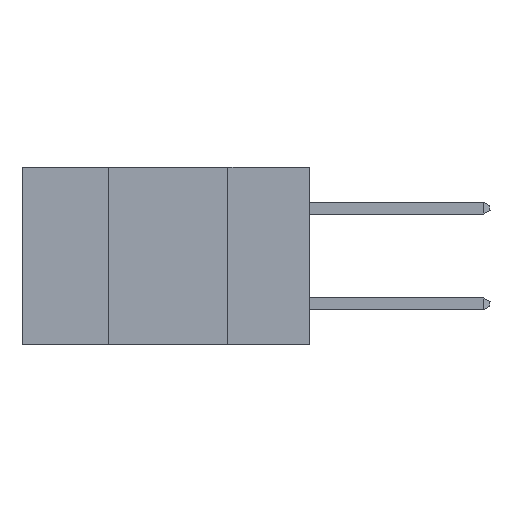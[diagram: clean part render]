
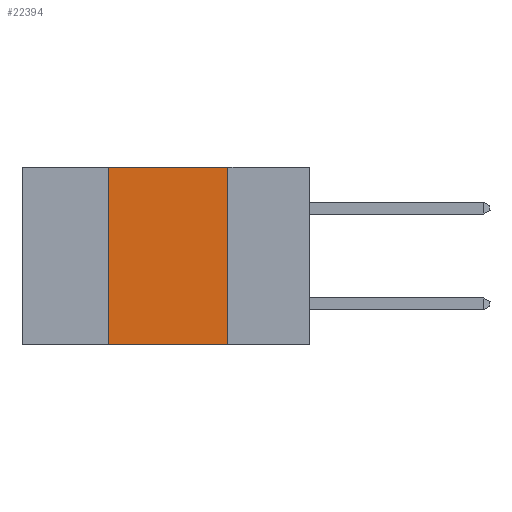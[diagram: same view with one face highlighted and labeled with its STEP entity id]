
A CAD part, left-side view. The second image highlights one B-rep face of the part: STEP entity #22394.
In plain terms, the highlighted planar face has unit normal (-1, 0, 0).
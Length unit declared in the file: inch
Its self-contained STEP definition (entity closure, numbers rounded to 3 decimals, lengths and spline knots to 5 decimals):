
#157 = LINE ( 'NONE', #28019, #7155 ) ;
#649 = EDGE_CURVE ( 'NONE', #26703, #19103, #25296, .T. ) ;
#2117 = DIRECTION ( 'NONE',  ( 0., 0., -1. ) ) ;
#2848 = LINE ( 'NONE', #33479, #21224 ) ;
#3149 = VERTEX_POINT ( 'NONE', #25572 ) ;
#4349 = DIRECTION ( 'NONE',  ( 0., -1., 0. ) ) ;
#6671 = CARTESIAN_POINT ( 'NONE',  ( 0., 0.6, -0.37 ) ) ;
#7155 = VECTOR ( 'NONE', #7980, 39.37008 ) ;
#7980 = DIRECTION ( 'NONE',  ( 0., 0., 1. ) ) ;
#8028 = FACE_OUTER_BOUND ( 'NONE', #17641, .T. ) ;
#10163 = PLANE ( 'NONE',  #22020 ) ;
#14916 = ORIENTED_EDGE ( 'NONE', *, *, #29927, .T. ) ;
#16187 = LINE ( 'NONE', #6671, #20147 ) ;
#17641 = EDGE_LOOP ( 'NONE', ( #25315, #28870, #25459, #14916 ) ) ;
#17831 = VECTOR ( 'NONE', #28814, 39.37008 ) ;
#18971 = CARTESIAN_POINT ( 'NONE',  ( 0., 0.6, 0. ) ) ;
#19103 = VERTEX_POINT ( 'NONE', #31976 ) ;
#19559 = DIRECTION ( 'NONE',  ( 0., 0., -1. ) ) ;
#20147 = VECTOR ( 'NONE', #4349, 39.37008 ) ;
#21224 = VECTOR ( 'NONE', #19559, 39.37008 ) ;
#22020 = AXIS2_PLACEMENT_3D ( 'NONE', #18971, #35276, #2117 ) ;
#22394 = ADVANCED_FACE ( 'NONE', ( #8028 ), #10163, .F. ) ;
#22551 = EDGE_CURVE ( 'NONE', #3149, #26703, #157, .T. ) ;
#24783 = CARTESIAN_POINT ( 'NONE',  ( 0., 0.6, 0. ) ) ;
#25296 = LINE ( 'NONE', #24783, #17831 ) ;
#25315 = ORIENTED_EDGE ( 'NONE', *, *, #33183, .F. ) ;
#25459 = ORIENTED_EDGE ( 'NONE', *, *, #22551, .F. ) ;
#25572 = CARTESIAN_POINT ( 'NONE',  ( 0., 0.42, -0.37 ) ) ;
#26703 = VERTEX_POINT ( 'NONE', #34579 ) ;
#28019 = CARTESIAN_POINT ( 'NONE',  ( 0., 0.42, 0. ) ) ;
#28814 = DIRECTION ( 'NONE',  ( 0., -1., 0. ) ) ;
#28870 = ORIENTED_EDGE ( 'NONE', *, *, #649, .F. ) ;
#29764 = VERTEX_POINT ( 'NONE', #33842 ) ;
#29927 = EDGE_CURVE ( 'NONE', #3149, #29764, #16187, .T. ) ;
#31976 = CARTESIAN_POINT ( 'NONE',  ( 0., 0.17, 0. ) ) ;
#33183 = EDGE_CURVE ( 'NONE', #19103, #29764, #2848, .T. ) ;
#33479 = CARTESIAN_POINT ( 'NONE',  ( 0., 0.17, 0. ) ) ;
#33842 = CARTESIAN_POINT ( 'NONE',  ( 0., 0.17, -0.37 ) ) ;
#34579 = CARTESIAN_POINT ( 'NONE',  ( 0., 0.42, 0. ) ) ;
#35276 = DIRECTION ( 'NONE',  ( 1., 0., 0. ) ) ;
